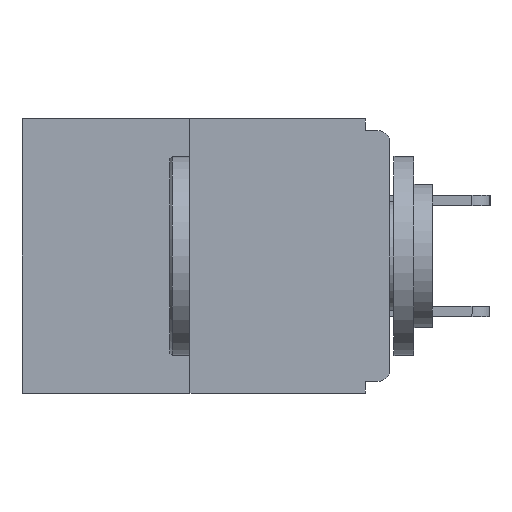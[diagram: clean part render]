
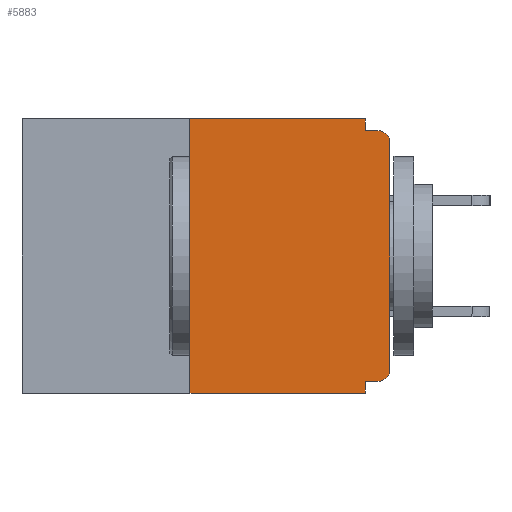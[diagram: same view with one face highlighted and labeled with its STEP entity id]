
A CAD part, left-side view. The second image highlights one B-rep face of the part: STEP entity #5883.
In plain terms, the highlighted planar face has unit normal (-1, 0, 0).
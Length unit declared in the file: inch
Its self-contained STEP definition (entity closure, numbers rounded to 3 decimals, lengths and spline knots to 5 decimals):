
#98 = CARTESIAN_POINT ( 'NONE',  ( 0., 0., -0.03 ) ) ;
#280 = LINE ( 'NONE', #24703, #13021 ) ;
#292 = CARTESIAN_POINT ( 'NONE',  ( 0., 0.25, 0. ) ) ;
#462 = CARTESIAN_POINT ( 'NONE',  ( 0., 0.015, -0.313 ) ) ;
#478 = CARTESIAN_POINT ( 'NONE',  ( 0., 0.25, -0.343 ) ) ;
#1172 = VERTEX_POINT ( 'NONE', #23067 ) ;
#1604 = AXIS2_PLACEMENT_3D ( 'NONE', #462, #2830, #21406 ) ;
#2830 = DIRECTION ( 'NONE',  ( -1., 0., 0. ) ) ;
#3121 = AXIS2_PLACEMENT_3D ( 'NONE', #7444, #20153, #3403 ) ;
#3222 = DIRECTION ( 'NONE',  ( 0., 0., 1. ) ) ;
#3403 = DIRECTION ( 'NONE',  ( 0., 0., -1. ) ) ;
#3767 = VECTOR ( 'NONE', #4921, 39.37008 ) ;
#3903 = DIRECTION ( 'NONE',  ( 0., 0., -1. ) ) ;
#4359 = EDGE_CURVE ( 'NONE', #12720, #1172, #280, .T. ) ;
#4666 = VECTOR ( 'NONE', #19765, 39.37008 ) ;
#4736 = CARTESIAN_POINT ( 'NONE',  ( 0., 0.46, -0.343 ) ) ;
#4811 = EDGE_CURVE ( 'NONE', #1172, #25219, #8601, .T. ) ;
#4921 = DIRECTION ( 'NONE',  ( 0., 0., -1. ) ) ;
#5883 = ADVANCED_FACE ( 'NONE', ( #22601 ), #17534, .F. ) ;
#5973 = CARTESIAN_POINT ( 'NONE',  ( 0., 0., -0.313 ) ) ;
#6033 = EDGE_CURVE ( 'NONE', #16231, #25463, #17381, .T. ) ;
#6202 = DIRECTION ( 'NONE',  ( -1., 0., 0. ) ) ;
#6477 = EDGE_CURVE ( 'NONE', #22203, #15090, #8838, .T. ) ;
#7091 = CARTESIAN_POINT ( 'NONE',  ( 0., 0.031, -0.343 ) ) ;
#7279 = CARTESIAN_POINT ( 'NONE',  ( 0., 0., 0. ) ) ;
#7444 = CARTESIAN_POINT ( 'NONE',  ( 0., 0.46, 0. ) ) ;
#7640 = CARTESIAN_POINT ( 'NONE',  ( 0., 0.015, -0.015 ) ) ;
#7687 = AXIS2_PLACEMENT_3D ( 'NONE', #14617, #6202, #3903 ) ;
#8256 = EDGE_LOOP ( 'NONE', ( #26358, #9425, #12533, #25981, #8955, #11005, #14599, #21234, #26490, #16988 ) ) ;
#8338 = DIRECTION ( 'NONE',  ( 0., -1., 0. ) ) ;
#8601 = LINE ( 'NONE', #7091, #16122 ) ;
#8838 = CIRCLE ( 'NONE', #7687, 0.015 ) ;
#8955 = ORIENTED_EDGE ( 'NONE', *, *, #4359, .F. ) ;
#9279 = LINE ( 'NONE', #7279, #13516 ) ;
#9365 = EDGE_CURVE ( 'NONE', #17739, #25219, #13561, .T. ) ;
#9425 = ORIENTED_EDGE ( 'NONE', *, *, #13820, .F. ) ;
#9511 = CARTESIAN_POINT ( 'NONE',  ( 0., 0., -0.015 ) ) ;
#9812 = VECTOR ( 'NONE', #8338, 39.37008 ) ;
#10216 = LINE ( 'NONE', #9511, #4666 ) ;
#11005 = ORIENTED_EDGE ( 'NONE', *, *, #26177, .T. ) ;
#12171 = DIRECTION ( 'NONE',  ( 0., 0., 1. ) ) ;
#12518 = CARTESIAN_POINT ( 'NONE',  ( 0., 0.46, 0. ) ) ;
#12533 = ORIENTED_EDGE ( 'NONE', *, *, #9365, .T. ) ;
#12720 = VERTEX_POINT ( 'NONE', #22893 ) ;
#13021 = VECTOR ( 'NONE', #14050, 39.37008 ) ;
#13516 = VECTOR ( 'NONE', #3222, 39.37008 ) ;
#13561 = LINE ( 'NONE', #4736, #20440 ) ;
#13820 = EDGE_CURVE ( 'NONE', #17739, #16231, #23489, .T. ) ;
#14050 = DIRECTION ( 'NONE',  ( 0., 1., 0. ) ) ;
#14599 = ORIENTED_EDGE ( 'NONE', *, *, #25063, .T. ) ;
#14617 = CARTESIAN_POINT ( 'NONE',  ( 0., 0.015, -0.03 ) ) ;
#14834 = CIRCLE ( 'NONE', #1604, 0.015 ) ;
#14988 = DIRECTION ( 'NONE',  ( 0., -1., 0. ) ) ;
#15090 = VERTEX_POINT ( 'NONE', #7640 ) ;
#15632 = CARTESIAN_POINT ( 'NONE',  ( 0., 0.031, 0. ) ) ;
#15856 = CARTESIAN_POINT ( 'NONE',  ( 0., 0.031, -0.343 ) ) ;
#16122 = VECTOR ( 'NONE', #19873, 39.37008 ) ;
#16231 = VERTEX_POINT ( 'NONE', #292 ) ;
#16306 = EDGE_CURVE ( 'NONE', #19937, #15090, #10216, .T. ) ;
#16988 = ORIENTED_EDGE ( 'NONE', *, *, #24196, .F. ) ;
#17381 = LINE ( 'NONE', #12518, #9812 ) ;
#17534 = PLANE ( 'NONE',  #3121 ) ;
#17739 = VERTEX_POINT ( 'NONE', #478 ) ;
#17847 = LINE ( 'NONE', #15632, #3767 ) ;
#17895 = VECTOR ( 'NONE', #12171, 39.37008 ) ;
#18249 = CARTESIAN_POINT ( 'NONE',  ( 0., 0.25, 0. ) ) ;
#18362 = VERTEX_POINT ( 'NONE', #5973 ) ;
#19765 = DIRECTION ( 'NONE',  ( 0., -1., 0. ) ) ;
#19873 = DIRECTION ( 'NONE',  ( 0., 0., -1. ) ) ;
#19937 = VERTEX_POINT ( 'NONE', #25825 ) ;
#20153 = DIRECTION ( 'NONE',  ( 1., 0., 0. ) ) ;
#20440 = VECTOR ( 'NONE', #14988, 39.37008 ) ;
#21052 = CARTESIAN_POINT ( 'NONE',  ( 0., 0.031, 0. ) ) ;
#21234 = ORIENTED_EDGE ( 'NONE', *, *, #6477, .T. ) ;
#21406 = DIRECTION ( 'NONE',  ( 0., 0., -1. ) ) ;
#22203 = VERTEX_POINT ( 'NONE', #98 ) ;
#22601 = FACE_OUTER_BOUND ( 'NONE', #8256, .T. ) ;
#22893 = CARTESIAN_POINT ( 'NONE',  ( 0., 0.015, -0.328 ) ) ;
#23067 = CARTESIAN_POINT ( 'NONE',  ( 0., 0.031, -0.328 ) ) ;
#23489 = LINE ( 'NONE', #18249, #17895 ) ;
#24196 = EDGE_CURVE ( 'NONE', #25463, #19937, #17847, .T. ) ;
#24703 = CARTESIAN_POINT ( 'NONE',  ( 0., 0., -0.328 ) ) ;
#25063 = EDGE_CURVE ( 'NONE', #18362, #22203, #9279, .T. ) ;
#25219 = VERTEX_POINT ( 'NONE', #15856 ) ;
#25463 = VERTEX_POINT ( 'NONE', #21052 ) ;
#25825 = CARTESIAN_POINT ( 'NONE',  ( 0., 0.031, -0.015 ) ) ;
#25981 = ORIENTED_EDGE ( 'NONE', *, *, #4811, .F. ) ;
#26177 = EDGE_CURVE ( 'NONE', #12720, #18362, #14834, .T. ) ;
#26358 = ORIENTED_EDGE ( 'NONE', *, *, #6033, .F. ) ;
#26490 = ORIENTED_EDGE ( 'NONE', *, *, #16306, .F. ) ;
